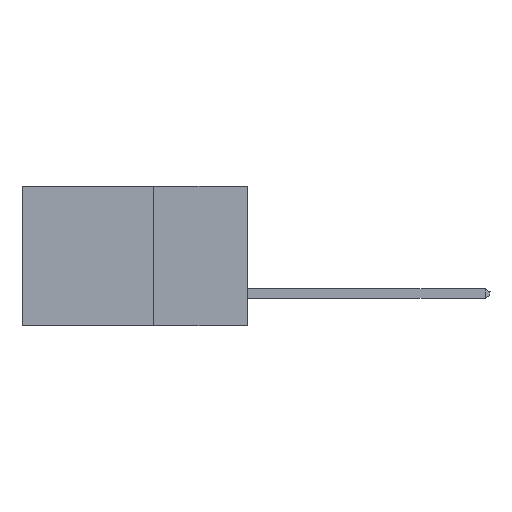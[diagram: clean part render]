
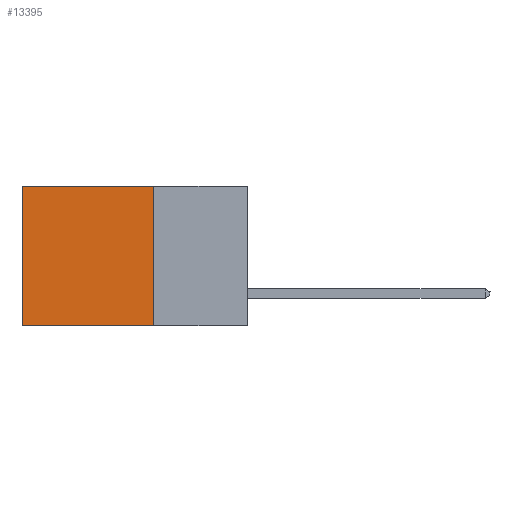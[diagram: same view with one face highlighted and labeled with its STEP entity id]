
A CAD part, left-side view. The second image highlights one B-rep face of the part: STEP entity #13395.
In plain terms, the highlighted planar face has unit normal (-1, 0, 0).
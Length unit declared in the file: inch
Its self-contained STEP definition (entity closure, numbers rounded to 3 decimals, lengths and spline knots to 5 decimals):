
#32 = FACE_OUTER_BOUND ( 'NONE', #7226, .T. ) ;
#163 = LINE ( 'NONE', #14204, #13089 ) ;
#1035 = VERTEX_POINT ( 'NONE', #5580 ) ;
#1382 = EDGE_CURVE ( 'NONE', #4482, #1035, #7801, .T. ) ;
#1724 = LINE ( 'NONE', #6773, #11029 ) ;
#2543 = VERTEX_POINT ( 'NONE', #9910 ) ;
#2877 = DIRECTION ( 'NONE',  ( 0., 1., 0. ) ) ;
#3806 = AXIS2_PLACEMENT_3D ( 'NONE', #6133, #9957, #7631 ) ;
#4005 = CARTESIAN_POINT ( 'NONE',  ( 0.2615, 0.25, 0. ) ) ;
#4482 = VERTEX_POINT ( 'NONE', #4005 ) ;
#5141 = VECTOR ( 'NONE', #6564, 39.37008 ) ;
#5457 = LINE ( 'NONE', #7026, #9110 ) ;
#5580 = CARTESIAN_POINT ( 'NONE',  ( 0.2615, 0.25, -0.37 ) ) ;
#5612 = DIRECTION ( 'NONE',  ( 0., 1., 0. ) ) ;
#5859 = ORIENTED_EDGE ( 'NONE', *, *, #8365, .F. ) ;
#5926 = ORIENTED_EDGE ( 'NONE', *, *, #1382, .F. ) ;
#6133 = CARTESIAN_POINT ( 'NONE',  ( 0.2615, 0.25, -0.37 ) ) ;
#6564 = DIRECTION ( 'NONE',  ( 0., 0., -1. ) ) ;
#6773 = CARTESIAN_POINT ( 'NONE',  ( 0.2615, 0.25, -0.37 ) ) ;
#6786 = CARTESIAN_POINT ( 'NONE',  ( 0.2615, 0.6, 0. ) ) ;
#7026 = CARTESIAN_POINT ( 'NONE',  ( 0.2615, 0.6, -0.37 ) ) ;
#7226 = EDGE_LOOP ( 'NONE', ( #9284, #5859, #5926, #12819 ) ) ;
#7631 = DIRECTION ( 'NONE',  ( 0., 0., -1. ) ) ;
#7801 = LINE ( 'NONE', #11599, #5141 ) ;
#8365 = EDGE_CURVE ( 'NONE', #1035, #2543, #1724, .T. ) ;
#9110 = VECTOR ( 'NONE', #12063, 39.37008 ) ;
#9284 = ORIENTED_EDGE ( 'NONE', *, *, #14644, .T. ) ;
#9910 = CARTESIAN_POINT ( 'NONE',  ( 0.2615, 0.6, -0.37 ) ) ;
#9957 = DIRECTION ( 'NONE',  ( 1., 0., 0. ) ) ;
#11029 = VECTOR ( 'NONE', #5612, 39.37008 ) ;
#11599 = CARTESIAN_POINT ( 'NONE',  ( 0.2615, 0.25, -0.37 ) ) ;
#12063 = DIRECTION ( 'NONE',  ( 0., 0., -1. ) ) ;
#12819 = ORIENTED_EDGE ( 'NONE', *, *, #16196, .T. ) ;
#13089 = VECTOR ( 'NONE', #2877, 39.37008 ) ;
#13395 = ADVANCED_FACE ( 'NONE', ( #32 ), #13898, .F. ) ;
#13898 = PLANE ( 'NONE',  #3806 ) ;
#14204 = CARTESIAN_POINT ( 'NONE',  ( 0.2615, 0.25, 0. ) ) ;
#14644 = EDGE_CURVE ( 'NONE', #15856, #2543, #5457, .T. ) ;
#15856 = VERTEX_POINT ( 'NONE', #6786 ) ;
#16196 = EDGE_CURVE ( 'NONE', #4482, #15856, #163, .T. ) ;
